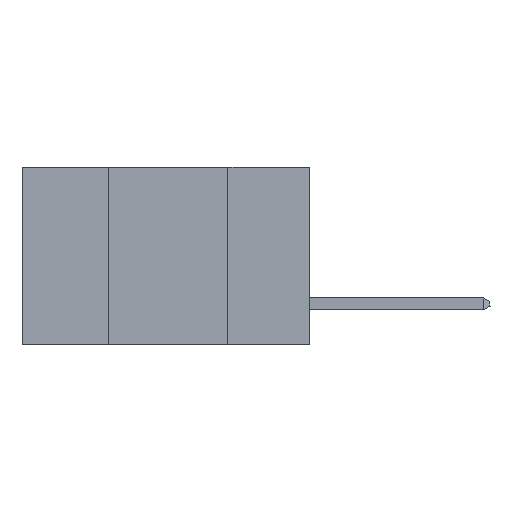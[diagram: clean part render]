
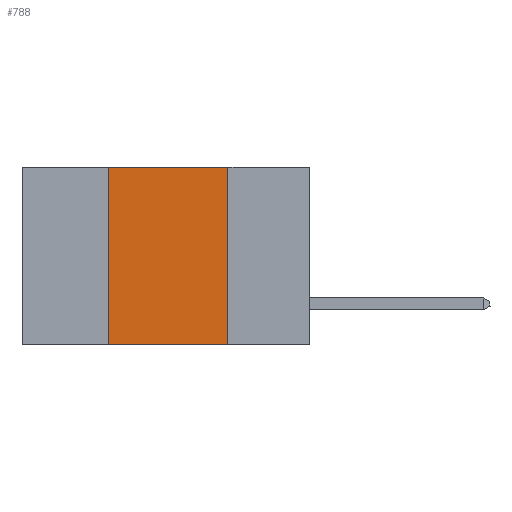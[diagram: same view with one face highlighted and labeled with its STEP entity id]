
A CAD part, left-side view. The second image highlights one B-rep face of the part: STEP entity #788.
In plain terms, the highlighted planar face has unit normal (-1, 0, 0).
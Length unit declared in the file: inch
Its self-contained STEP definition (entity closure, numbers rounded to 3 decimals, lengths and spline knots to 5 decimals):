
#786 = PLANE ( 'NONE',  #9111 ) ;
#788 = ADVANCED_FACE ( 'NONE', ( #12440 ), #786, .F. ) ;
#1027 = DIRECTION ( 'NONE',  ( 0., -1., 0. ) ) ;
#1157 = EDGE_LOOP ( 'NONE', ( #12184, #4071, #20639, #12667 ) ) ;
#2267 = VECTOR ( 'NONE', #10420, 39.37008 ) ;
#2455 = DIRECTION ( 'NONE',  ( 0., 0., -1. ) ) ;
#3044 = LINE ( 'NONE', #10944, #16912 ) ;
#4071 = ORIENTED_EDGE ( 'NONE', *, *, #4332, .F. ) ;
#4332 = EDGE_CURVE ( 'NONE', #4642, #8406, #3044, .T. ) ;
#4642 = VERTEX_POINT ( 'NONE', #17388 ) ;
#5241 = VERTEX_POINT ( 'NONE', #18298 ) ;
#6906 = CARTESIAN_POINT ( 'NONE',  ( 0., 0.42, 0. ) ) ;
#7437 = LINE ( 'NONE', #13450, #13307 ) ;
#7694 = LINE ( 'NONE', #6906, #2267 ) ;
#8406 = VERTEX_POINT ( 'NONE', #20857 ) ;
#9111 = AXIS2_PLACEMENT_3D ( 'NONE', #20276, #12273, #2455 ) ;
#10420 = DIRECTION ( 'NONE',  ( 0., 0., 1. ) ) ;
#10944 = CARTESIAN_POINT ( 'NONE',  ( 0., 0.6, 0. ) ) ;
#12184 = ORIENTED_EDGE ( 'NONE', *, *, #16115, .F. ) ;
#12273 = DIRECTION ( 'NONE',  ( 1., 0., 0. ) ) ;
#12440 = FACE_OUTER_BOUND ( 'NONE', #1157, .T. ) ;
#12667 = ORIENTED_EDGE ( 'NONE', *, *, #12956, .T. ) ;
#12956 = EDGE_CURVE ( 'NONE', #16098, #5241, #16248, .T. ) ;
#13307 = VECTOR ( 'NONE', #15033, 39.37008 ) ;
#13450 = CARTESIAN_POINT ( 'NONE',  ( 0., 0.17, 0. ) ) ;
#13669 = CARTESIAN_POINT ( 'NONE',  ( 0., 0.42, -0.37 ) ) ;
#13848 = CARTESIAN_POINT ( 'NONE',  ( 0., 0.6, -0.37 ) ) ;
#15033 = DIRECTION ( 'NONE',  ( 0., 0., -1. ) ) ;
#16098 = VERTEX_POINT ( 'NONE', #13669 ) ;
#16115 = EDGE_CURVE ( 'NONE', #8406, #5241, #7437, .T. ) ;
#16248 = LINE ( 'NONE', #13848, #18081 ) ;
#16912 = VECTOR ( 'NONE', #1027, 39.37008 ) ;
#17388 = CARTESIAN_POINT ( 'NONE',  ( 0., 0.42, 0. ) ) ;
#18081 = VECTOR ( 'NONE', #20220, 39.37008 ) ;
#18298 = CARTESIAN_POINT ( 'NONE',  ( 0., 0.17, -0.37 ) ) ;
#20220 = DIRECTION ( 'NONE',  ( 0., -1., 0. ) ) ;
#20276 = CARTESIAN_POINT ( 'NONE',  ( 0., 0.6, 0. ) ) ;
#20639 = ORIENTED_EDGE ( 'NONE', *, *, #21038, .F. ) ;
#20857 = CARTESIAN_POINT ( 'NONE',  ( 0., 0.17, 0. ) ) ;
#21038 = EDGE_CURVE ( 'NONE', #16098, #4642, #7694, .T. ) ;
